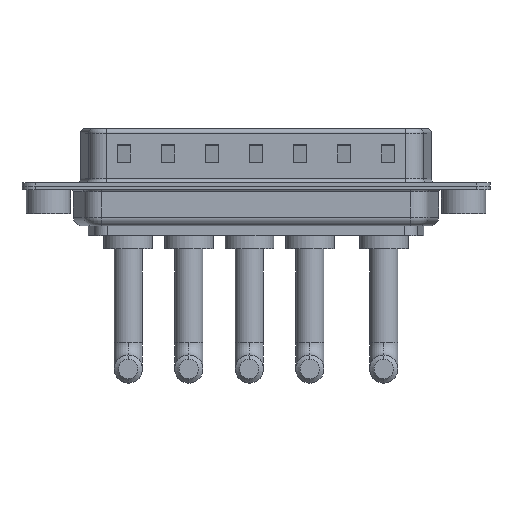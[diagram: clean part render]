
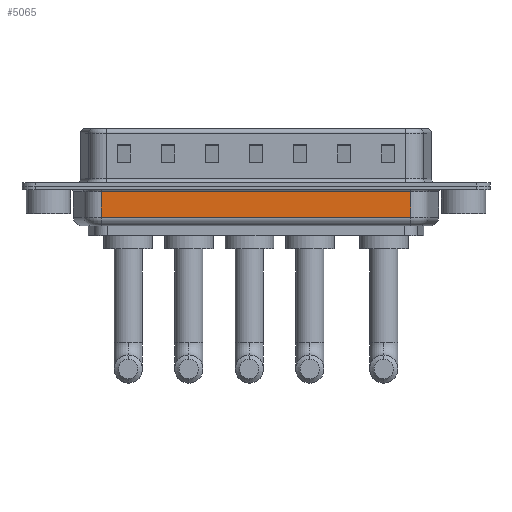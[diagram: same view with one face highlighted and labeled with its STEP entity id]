
A CAD part, front view. The second image highlights one B-rep face of the part: STEP entity #5065.
In plain terms, the highlighted planar face has unit normal (0, -1, 0).
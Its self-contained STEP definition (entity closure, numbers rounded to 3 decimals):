
#91 = CARTESIAN_POINT ( 'NONE',  ( 6.006, -5.35, -4.5 ) ) ;
#489 = LINE ( 'NONE', #6966, #7221 ) ;
#2021 = EDGE_CURVE ( 'NONE', #12018, #11134, #14039, .T. ) ;
#2299 = LINE ( 'NONE', #12229, #4713 ) ;
#2402 = DIRECTION ( 'NONE',  ( 0., 0., 1. ) ) ;
#2807 = VECTOR ( 'NONE', #7305, 1000. ) ;
#3009 = CARTESIAN_POINT ( 'NONE',  ( 41.044, -5.35, -4.5 ) ) ;
#3127 = ORIENTED_EDGE ( 'NONE', *, *, #6953, .T. ) ;
#3447 = DIRECTION ( 'NONE',  ( 0., 0., 1. ) ) ;
#3609 = VERTEX_POINT ( 'NONE', #9282 ) ;
#4021 = ORIENTED_EDGE ( 'NONE', *, *, #11820, .T. ) ;
#4423 = DIRECTION ( 'NONE',  ( 1., 0., 0. ) ) ;
#4545 = DIRECTION ( 'NONE',  ( 0., 1., 0. ) ) ;
#4713 = VECTOR ( 'NONE', #6721, 1000. ) ;
#5065 = ADVANCED_FACE ( 'NONE', ( #12066 ), #10097, .F. ) ;
#5520 = AXIS2_PLACEMENT_3D ( 'NONE', #91, #4545, #3447 ) ;
#5751 = EDGE_LOOP ( 'NONE', ( #13660, #3127, #9324, #4021 ) ) ;
#6721 = DIRECTION ( 'NONE',  ( -1., 0., 0. ) ) ;
#6730 = CARTESIAN_POINT ( 'NONE',  ( 6.006, -5.35, -3.5 ) ) ;
#6953 = EDGE_CURVE ( 'NONE', #9717, #12018, #14421, .T. ) ;
#6966 = CARTESIAN_POINT ( 'NONE',  ( 6.006, -5.35, -4.5 ) ) ;
#7221 = VECTOR ( 'NONE', #2402, 1000. ) ;
#7305 = DIRECTION ( 'NONE',  ( 0., 0., 1. ) ) ;
#7516 = CARTESIAN_POINT ( 'NONE',  ( 6.006, -5.35, -3.5 ) ) ;
#8496 = EDGE_CURVE ( 'NONE', #9717, #3609, #489, .T. ) ;
#8738 = CARTESIAN_POINT ( 'NONE',  ( 41.044, -5.35, -0.65 ) ) ;
#9282 = CARTESIAN_POINT ( 'NONE',  ( 6.006, -5.35, -0.65 ) ) ;
#9324 = ORIENTED_EDGE ( 'NONE', *, *, #2021, .T. ) ;
#9717 = VERTEX_POINT ( 'NONE', #7516 ) ;
#10097 = PLANE ( 'NONE',  #5520 ) ;
#11134 = VERTEX_POINT ( 'NONE', #8738 ) ;
#11820 = EDGE_CURVE ( 'NONE', #11134, #3609, #2299, .T. ) ;
#12018 = VERTEX_POINT ( 'NONE', #13517 ) ;
#12066 = FACE_OUTER_BOUND ( 'NONE', #5751, .T. ) ;
#12162 = VECTOR ( 'NONE', #4423, 1000. ) ;
#12229 = CARTESIAN_POINT ( 'NONE',  ( 6.006, -5.35, -0.65 ) ) ;
#13517 = CARTESIAN_POINT ( 'NONE',  ( 41.044, -5.35, -3.5 ) ) ;
#13660 = ORIENTED_EDGE ( 'NONE', *, *, #8496, .F. ) ;
#14039 = LINE ( 'NONE', #3009, #2807 ) ;
#14421 = LINE ( 'NONE', #6730, #12162 ) ;
